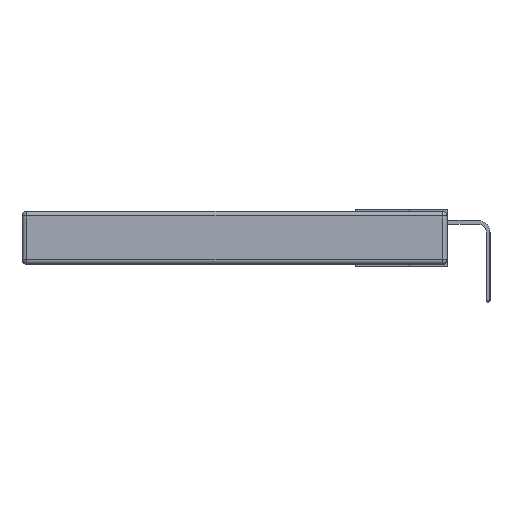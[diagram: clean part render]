
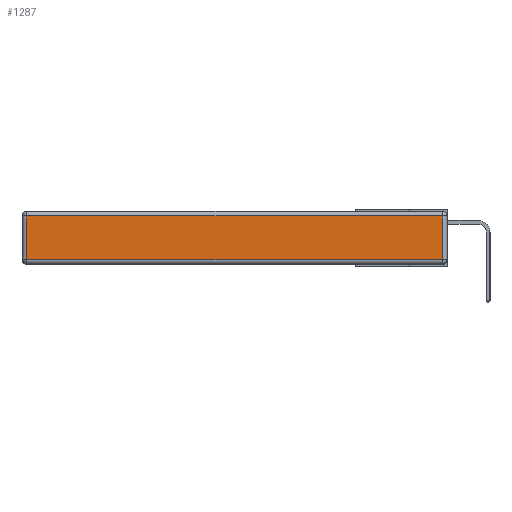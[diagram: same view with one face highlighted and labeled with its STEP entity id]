
A CAD part, left-side view. The second image highlights one B-rep face of the part: STEP entity #1287.
In plain terms, the highlighted planar face has unit normal (-1, 0, 0).
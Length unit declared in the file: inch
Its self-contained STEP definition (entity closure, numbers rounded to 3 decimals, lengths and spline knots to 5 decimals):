
#155 = VECTOR ( 'NONE', #15805, 39.37008 ) ;
#489 = CARTESIAN_POINT ( 'NONE',  ( 0., 0.03, -0.343 ) ) ;
#741 = ORIENTED_EDGE ( 'NONE', *, *, #7302, .T. ) ;
#1287 = ADVANCED_FACE ( 'NONE', ( #20515 ), #5229, .T. ) ;
#2403 = LINE ( 'NONE', #16921, #23196 ) ;
#2609 = VECTOR ( 'NONE', #14634, 39.37008 ) ;
#3399 = CARTESIAN_POINT ( 'NONE',  ( 0., 0.03, -0.313 ) ) ;
#3999 = LINE ( 'NONE', #12913, #24441 ) ;
#5229 = PLANE ( 'NONE',  #16727 ) ;
#5416 = CARTESIAN_POINT ( 'NONE',  ( 0., 0.03, -0.03 ) ) ;
#5858 = ORIENTED_EDGE ( 'NONE', *, *, #23961, .T. ) ;
#6324 = VERTEX_POINT ( 'NONE', #3399 ) ;
#6492 = LINE ( 'NONE', #13812, #155 ) ;
#7302 = EDGE_CURVE ( 'NONE', #15063, #8829, #6492, .T. ) ;
#8599 = EDGE_CURVE ( 'NONE', #6324, #15063, #25263, .T. ) ;
#8829 = VERTEX_POINT ( 'NONE', #23230 ) ;
#8924 = DIRECTION ( 'NONE',  ( 0., -1., 0. ) ) ;
#11238 = DIRECTION ( 'NONE',  ( 0., 0., 1. ) ) ;
#12002 = ORIENTED_EDGE ( 'NONE', *, *, #8599, .T. ) ;
#12913 = CARTESIAN_POINT ( 'NONE',  ( 0., 0., -0.313 ) ) ;
#13812 = CARTESIAN_POINT ( 'NONE',  ( 0., 2.75, -0.03 ) ) ;
#14634 = DIRECTION ( 'NONE',  ( 0., 0., 1. ) ) ;
#15063 = VERTEX_POINT ( 'NONE', #5416 ) ;
#15805 = DIRECTION ( 'NONE',  ( 0., 1., 0. ) ) ;
#15868 = VERTEX_POINT ( 'NONE', #23455 ) ;
#16727 = AXIS2_PLACEMENT_3D ( 'NONE', #21246, #25089, #11238 ) ;
#16921 = CARTESIAN_POINT ( 'NONE',  ( 0., 2.72, -0.343 ) ) ;
#17003 = DIRECTION ( 'NONE',  ( 0., 0., -1. ) ) ;
#20515 = FACE_OUTER_BOUND ( 'NONE', #25821, .T. ) ;
#20916 = ORIENTED_EDGE ( 'NONE', *, *, #23991, .T. ) ;
#21246 = CARTESIAN_POINT ( 'NONE',  ( 0., 0., -0.343 ) ) ;
#23196 = VECTOR ( 'NONE', #17003, 39.37008 ) ;
#23230 = CARTESIAN_POINT ( 'NONE',  ( 0., 2.72, -0.03 ) ) ;
#23455 = CARTESIAN_POINT ( 'NONE',  ( 0., 2.72, -0.313 ) ) ;
#23961 = EDGE_CURVE ( 'NONE', #15868, #6324, #3999, .T. ) ;
#23991 = EDGE_CURVE ( 'NONE', #8829, #15868, #2403, .T. ) ;
#24441 = VECTOR ( 'NONE', #8924, 39.37008 ) ;
#25089 = DIRECTION ( 'NONE',  ( -1., 0., 0. ) ) ;
#25263 = LINE ( 'NONE', #489, #2609 ) ;
#25821 = EDGE_LOOP ( 'NONE', ( #5858, #12002, #741, #20916 ) ) ;
